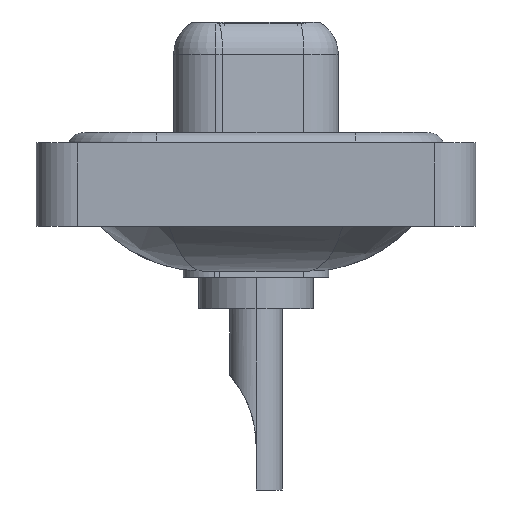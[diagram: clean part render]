
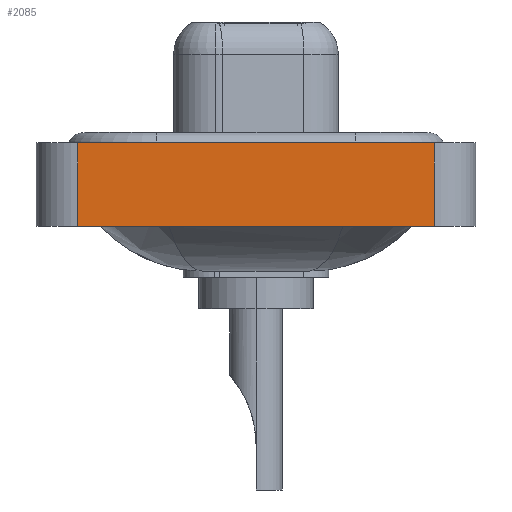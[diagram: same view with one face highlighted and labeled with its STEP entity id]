
A CAD part, left-side view. The second image highlights one B-rep face of the part: STEP entity #2085.
In plain terms, the highlighted planar face has unit normal (-1, 0, 0).
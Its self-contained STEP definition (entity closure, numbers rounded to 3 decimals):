
#213 = VECTOR ( 'NONE', #14485, 1000. ) ;
#1042 = VERTEX_POINT ( 'NONE', #5618 ) ;
#2085 = ADVANCED_FACE ( 'NONE', ( #7542 ), #13479, .T. ) ;
#2528 = CARTESIAN_POINT ( 'NONE',  ( -7.25, -8.55, -3.6 ) ) ;
#3050 = CARTESIAN_POINT ( 'NONE',  ( -7.25, -8.55, -3.6 ) ) ;
#3364 = VERTEX_POINT ( 'NONE', #10471 ) ;
#3872 = DIRECTION ( 'NONE',  ( -1., 0., 0. ) ) ;
#4016 = VECTOR ( 'NONE', #12614, 1000. ) ;
#4179 = AXIS2_PLACEMENT_3D ( 'NONE', #2528, #3872, #11068 ) ;
#4288 = VECTOR ( 'NONE', #12049, 1000. ) ;
#4340 = LINE ( 'NONE', #6808, #15723 ) ;
#4492 = EDGE_LOOP ( 'NONE', ( #5916, #15265, #10246, #4543 ) ) ;
#4543 = ORIENTED_EDGE ( 'NONE', *, *, #12235, .T. ) ;
#5618 = CARTESIAN_POINT ( 'NONE',  ( -7.25, -8.55, 0.4 ) ) ;
#5849 = EDGE_CURVE ( 'NONE', #6086, #1042, #5850, .T. ) ;
#5850 = LINE ( 'NONE', #10730, #213 ) ;
#5916 = ORIENTED_EDGE ( 'NONE', *, *, #5849, .T. ) ;
#6086 = VERTEX_POINT ( 'NONE', #3050 ) ;
#6526 = LINE ( 'NONE', #13814, #4016 ) ;
#6808 = CARTESIAN_POINT ( 'NONE',  ( -7.25, -8.55, 0.4 ) ) ;
#7542 = FACE_OUTER_BOUND ( 'NONE', #4492, .T. ) ;
#8710 = EDGE_CURVE ( 'NONE', #3364, #1042, #4340, .T. ) ;
#10246 = ORIENTED_EDGE ( 'NONE', *, *, #12478, .F. ) ;
#10471 = CARTESIAN_POINT ( 'NONE',  ( -7.25, 8.55, 0.4 ) ) ;
#10730 = CARTESIAN_POINT ( 'NONE',  ( -7.25, -8.55, -3.6 ) ) ;
#10805 = VERTEX_POINT ( 'NONE', #11084 ) ;
#10837 = CARTESIAN_POINT ( 'NONE',  ( -7.25, 8.55, -3.6 ) ) ;
#11068 = DIRECTION ( 'NONE',  ( 0., 0., 1. ) ) ;
#11084 = CARTESIAN_POINT ( 'NONE',  ( -7.25, 8.55, -3.6 ) ) ;
#11694 = DIRECTION ( 'NONE',  ( 0., -1., 0. ) ) ;
#12049 = DIRECTION ( 'NONE',  ( 0., 0., 1. ) ) ;
#12235 = EDGE_CURVE ( 'NONE', #10805, #6086, #6526, .T. ) ;
#12478 = EDGE_CURVE ( 'NONE', #10805, #3364, #15570, .T. ) ;
#12614 = DIRECTION ( 'NONE',  ( 0., -1., 0. ) ) ;
#13479 = PLANE ( 'NONE',  #4179 ) ;
#13814 = CARTESIAN_POINT ( 'NONE',  ( -7.25, -8.55, -3.6 ) ) ;
#14485 = DIRECTION ( 'NONE',  ( 0., 0., 1. ) ) ;
#15265 = ORIENTED_EDGE ( 'NONE', *, *, #8710, .F. ) ;
#15570 = LINE ( 'NONE', #10837, #4288 ) ;
#15723 = VECTOR ( 'NONE', #11694, 1000. ) ;
